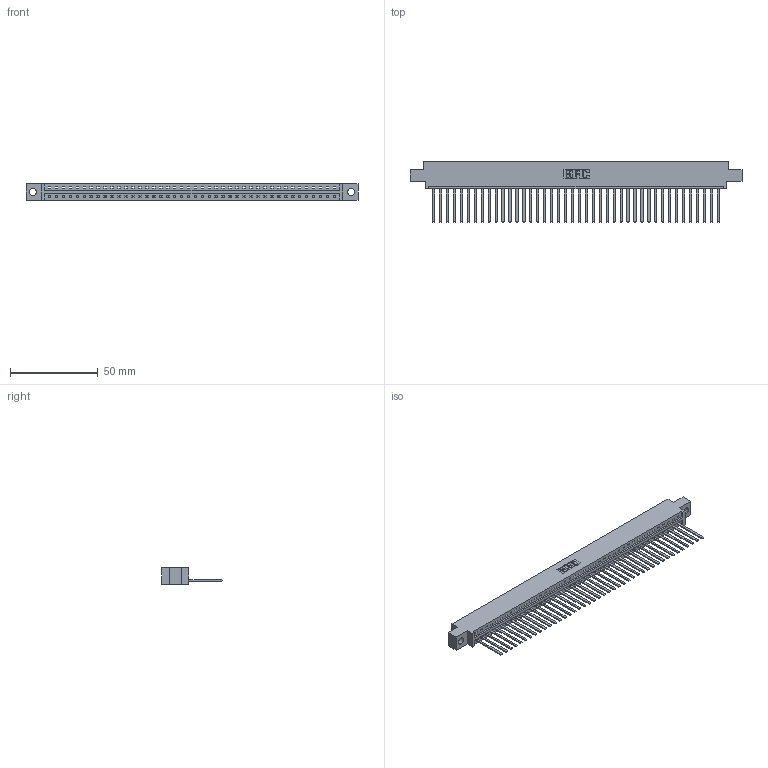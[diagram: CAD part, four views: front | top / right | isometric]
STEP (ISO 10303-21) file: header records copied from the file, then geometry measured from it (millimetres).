
FILE_DESCRIPTION (( 'STEP AP203' ), '1' );
FILE_NAME ('387-042-544-604.STEP', '2019-10-04T21:24:53', ( '' ), ( '' ), 'SwSTEP 2.0', 'SolidWorks 2016', '' );
FILE_SCHEMA (( 'CONFIG_CONTROL_DESIGN' ));
Length unit declared in the file: inch
Products named in the file (3): 345-292-001_345-293-144; 387-042-544-604; 337 Part_0.170 Offset - 0.156 Dia-TH
Assembly tree (43 placements, depth 2):
  387-042-544-604
    337 Part_0.170 Offset - 0.156 Dia-TH
    345-292-001_345-293-144  x42
Bounding box: 189.43 x 34.3 x 9.4 mm (x, y, z)
Volume: 19969.5 mm3; surface area: 22127.3 mm2
Topology: 43 solids, 43 shells, 2470 faces, 7463 edges, 4918 vertices
Faces by surface type: plane 1838, cylinder 632
Entity records: 31171 total; most frequent: CARTESIAN_POINT 5436, ORIENTED_EDGE 5414, DIRECTION 4571, EDGE_CURVE 2707, VECTOR 2583, LINE 2583, VERTEX_POINT 1802, AXIS2_PLACEMENT_3D 994
